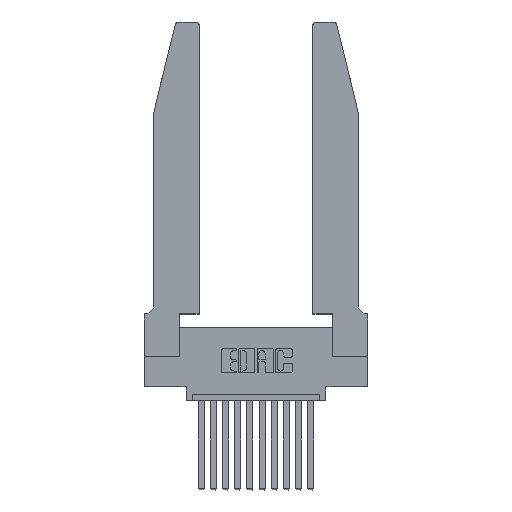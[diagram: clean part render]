
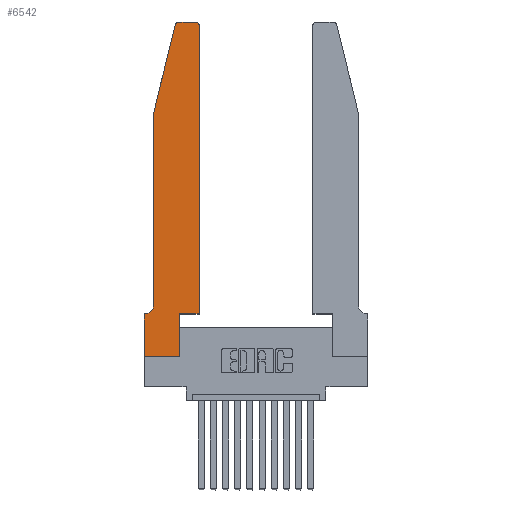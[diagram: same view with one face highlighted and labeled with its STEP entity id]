
A CAD part, top view. The second image highlights one B-rep face of the part: STEP entity #6542.
In plain terms, the highlighted planar face has unit normal (0, 0, 1).
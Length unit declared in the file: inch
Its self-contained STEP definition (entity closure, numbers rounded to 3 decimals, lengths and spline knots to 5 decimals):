
#610 = VERTEX_POINT ( 'NONE', #12630 ) ;
#801 = CARTESIAN_POINT ( 'NONE',  ( 0.4505, 0.35, 0.37 ) ) ;
#950 = DIRECTION ( 'NONE',  ( -0.239, -0.971, 0. ) ) ;
#1368 = EDGE_CURVE ( 'NONE', #4863, #11231, #15651, .T. ) ;
#1726 = LINE ( 'NONE', #15007, #8522 ) ;
#1824 = CARTESIAN_POINT ( 'NONE',  ( 0.2605, 2.75, 0.37 ) ) ;
#1857 = CARTESIAN_POINT ( 'NONE',  ( 0.4505, 2.72, 0.37 ) ) ;
#1872 = LINE ( 'NONE', #1824, #15021 ) ;
#2031 = EDGE_CURVE ( 'NONE', #6451, #4863, #12831, .T. ) ;
#2187 = VERTEX_POINT ( 'NONE', #4458 ) ;
#2234 = EDGE_CURVE ( 'NONE', #610, #16270, #1872, .T. ) ;
#2329 = LINE ( 'NONE', #15647, #4523 ) ;
#2685 = DIRECTION ( 'NONE',  ( 1., 0., 0. ) ) ;
#3080 = VECTOR ( 'NONE', #15421, 39.37008 ) ;
#3296 = LINE ( 'NONE', #13568, #6262 ) ;
#3344 = DIRECTION ( 'NONE',  ( 0., -1., 0. ) ) ;
#3444 = DIRECTION ( 'NONE',  ( 0., 0., 1. ) ) ;
#3446 = LINE ( 'NONE', #7631, #13985 ) ;
#3798 = ORIENTED_EDGE ( 'NONE', *, *, #6742, .T. ) ;
#3921 = DIRECTION ( 'NONE',  ( 0., 0., 1. ) ) ;
#3950 = CARTESIAN_POINT ( 'NONE',  ( 0.2865, 0., 0.37 ) ) ;
#4221 = CARTESIAN_POINT ( 'NONE',  ( 0., 0., 0.37 ) ) ;
#4311 = VERTEX_POINT ( 'NONE', #1857 ) ;
#4458 = CARTESIAN_POINT ( 'NONE',  ( 0.0755, 2., 0.37 ) ) ;
#4523 = VECTOR ( 'NONE', #12962, 39.37008 ) ;
#4531 = EDGE_CURVE ( 'NONE', #11231, #4311, #3446, .T. ) ;
#4571 = ORIENTED_EDGE ( 'NONE', *, *, #9361, .T. ) ;
#4575 = DIRECTION ( 'NONE',  ( 1., 0., 0. ) ) ;
#4742 = CARTESIAN_POINT ( 'NONE',  ( 0.0755, 0.42, 0.37 ) ) ;
#4863 = VERTEX_POINT ( 'NONE', #6101 ) ;
#5083 = ORIENTED_EDGE ( 'NONE', *, *, #4531, .T. ) ;
#5137 = LINE ( 'NONE', #4221, #13509 ) ;
#5542 = VERTEX_POINT ( 'NONE', #10105 ) ;
#5844 = DIRECTION ( 'NONE',  ( 1., 0., 0. ) ) ;
#5999 = CIRCLE ( 'NONE', #8656, 0.07 ) ;
#6081 = ORIENTED_EDGE ( 'NONE', *, *, #1368, .T. ) ;
#6082 = PLANE ( 'NONE',  #6211 ) ;
#6101 = CARTESIAN_POINT ( 'NONE',  ( 0.2865, 0.35, 0.37 ) ) ;
#6211 = AXIS2_PLACEMENT_3D ( 'NONE', #14990, #3921, #2685 ) ;
#6262 = VECTOR ( 'NONE', #3344, 39.37008 ) ;
#6451 = VERTEX_POINT ( 'NONE', #3950 ) ;
#6524 = CARTESIAN_POINT ( 'NONE',  ( 0.2865, 0.35, 0.37 ) ) ;
#6542 = ADVANCED_FACE ( 'NONE', ( #7974 ), #6082, .T. ) ;
#6742 = EDGE_CURVE ( 'NONE', #4311, #610, #9369, .T. ) ;
#7089 = EDGE_LOOP ( 'NONE', ( #11090, #11769, #16174, #12075, #8160, #8450, #4571, #8565, #11880, #6081, #5083, #3798 ) ) ;
#7305 = CIRCLE ( 'NONE', #10551, 0.03 ) ;
#7612 = VERTEX_POINT ( 'NONE', #4742 ) ;
#7631 = CARTESIAN_POINT ( 'NONE',  ( 0.4505, 0.35, 0.37 ) ) ;
#7974 = FACE_OUTER_BOUND ( 'NONE', #7089, .T. ) ;
#8160 = ORIENTED_EDGE ( 'NONE', *, *, #11799, .T. ) ;
#8444 = EDGE_CURVE ( 'NONE', #8636, #13160, #2329, .T. ) ;
#8450 = ORIENTED_EDGE ( 'NONE', *, *, #8444, .T. ) ;
#8522 = VECTOR ( 'NONE', #950, 39.37008 ) ;
#8565 = ORIENTED_EDGE ( 'NONE', *, *, #13721, .T. ) ;
#8636 = VERTEX_POINT ( 'NONE', #14240 ) ;
#8656 = AXIS2_PLACEMENT_3D ( 'NONE', #14766, #11217, #14820 ) ;
#8699 = AXIS2_PLACEMENT_3D ( 'NONE', #15873, #13472, #5844 ) ;
#8894 = VECTOR ( 'NONE', #9667, 39.37008 ) ;
#9106 = LINE ( 'NONE', #16249, #8894 ) ;
#9361 = EDGE_CURVE ( 'NONE', #13160, #14322, #3296, .T. ) ;
#9369 = CIRCLE ( 'NONE', #8699, 0.03 ) ;
#9389 = EDGE_CURVE ( 'NONE', #2187, #7612, #9106, .T. ) ;
#9667 = DIRECTION ( 'NONE',  ( 0., -1., 0. ) ) ;
#9962 = CARTESIAN_POINT ( 'NONE',  ( 0.284, 2.72, 0.37 ) ) ;
#10105 = CARTESIAN_POINT ( 'NONE',  ( 0.25487, 2.72718, 0.37 ) ) ;
#10551 = AXIS2_PLACEMENT_3D ( 'NONE', #9962, #3444, #16239 ) ;
#11060 = CARTESIAN_POINT ( 'NONE',  ( 0., 0., 0.37 ) ) ;
#11090 = ORIENTED_EDGE ( 'NONE', *, *, #2234, .T. ) ;
#11217 = DIRECTION ( 'NONE',  ( 0., 0., -1. ) ) ;
#11231 = VERTEX_POINT ( 'NONE', #11434 ) ;
#11434 = CARTESIAN_POINT ( 'NONE',  ( 0.4505, 0.35, 0.37 ) ) ;
#11769 = ORIENTED_EDGE ( 'NONE', *, *, #15041, .T. ) ;
#11799 = EDGE_CURVE ( 'NONE', #7612, #8636, #5999, .T. ) ;
#11880 = ORIENTED_EDGE ( 'NONE', *, *, #2031, .T. ) ;
#11980 = CARTESIAN_POINT ( 'NONE',  ( 0., 0.35, 0.37 ) ) ;
#12075 = ORIENTED_EDGE ( 'NONE', *, *, #9389, .T. ) ;
#12405 = DIRECTION ( 'NONE',  ( -1., 0., 0. ) ) ;
#12630 = CARTESIAN_POINT ( 'NONE',  ( 0.4205, 2.75, 0.37 ) ) ;
#12658 = DIRECTION ( 'NONE',  ( 0., 1., 0. ) ) ;
#12831 = LINE ( 'NONE', #6524, #3080 ) ;
#12962 = DIRECTION ( 'NONE',  ( -1., 0., 0. ) ) ;
#13160 = VERTEX_POINT ( 'NONE', #11980 ) ;
#13472 = DIRECTION ( 'NONE',  ( 0., 0., 1. ) ) ;
#13509 = VECTOR ( 'NONE', #14408, 39.37008 ) ;
#13568 = CARTESIAN_POINT ( 'NONE',  ( 0., 0., 0.37 ) ) ;
#13721 = EDGE_CURVE ( 'NONE', #14322, #6451, #5137, .T. ) ;
#13900 = CARTESIAN_POINT ( 'NONE',  ( 0.284, 2.75, 0.37 ) ) ;
#13931 = EDGE_CURVE ( 'NONE', #5542, #2187, #1726, .T. ) ;
#13985 = VECTOR ( 'NONE', #12658, 39.37008 ) ;
#14240 = CARTESIAN_POINT ( 'NONE',  ( 0.0055, 0.35, 0.37 ) ) ;
#14322 = VERTEX_POINT ( 'NONE', #11060 ) ;
#14408 = DIRECTION ( 'NONE',  ( 1., 0., 0. ) ) ;
#14766 = CARTESIAN_POINT ( 'NONE',  ( 0.0055, 0.42, 0.37 ) ) ;
#14820 = DIRECTION ( 'NONE',  ( -1., 0., 0. ) ) ;
#14847 = VECTOR ( 'NONE', #4575, 39.37008 ) ;
#14990 = CARTESIAN_POINT ( 'NONE',  ( 0., 0.35, 0.37 ) ) ;
#15007 = CARTESIAN_POINT ( 'NONE',  ( 0.0755, 2., 0.37 ) ) ;
#15021 = VECTOR ( 'NONE', #12405, 39.37008 ) ;
#15041 = EDGE_CURVE ( 'NONE', #16270, #5542, #7305, .T. ) ;
#15421 = DIRECTION ( 'NONE',  ( 0., 1., 0. ) ) ;
#15647 = CARTESIAN_POINT ( 'NONE',  ( 0.0755, 0.35, 0.37 ) ) ;
#15651 = LINE ( 'NONE', #801, #14847 ) ;
#15873 = CARTESIAN_POINT ( 'NONE',  ( 0.4205, 2.72, 0.37 ) ) ;
#16174 = ORIENTED_EDGE ( 'NONE', *, *, #13931, .T. ) ;
#16239 = DIRECTION ( 'NONE',  ( 1., 0., 0. ) ) ;
#16249 = CARTESIAN_POINT ( 'NONE',  ( 0.0755, 2., 0.37 ) ) ;
#16270 = VERTEX_POINT ( 'NONE', #13900 ) ;
